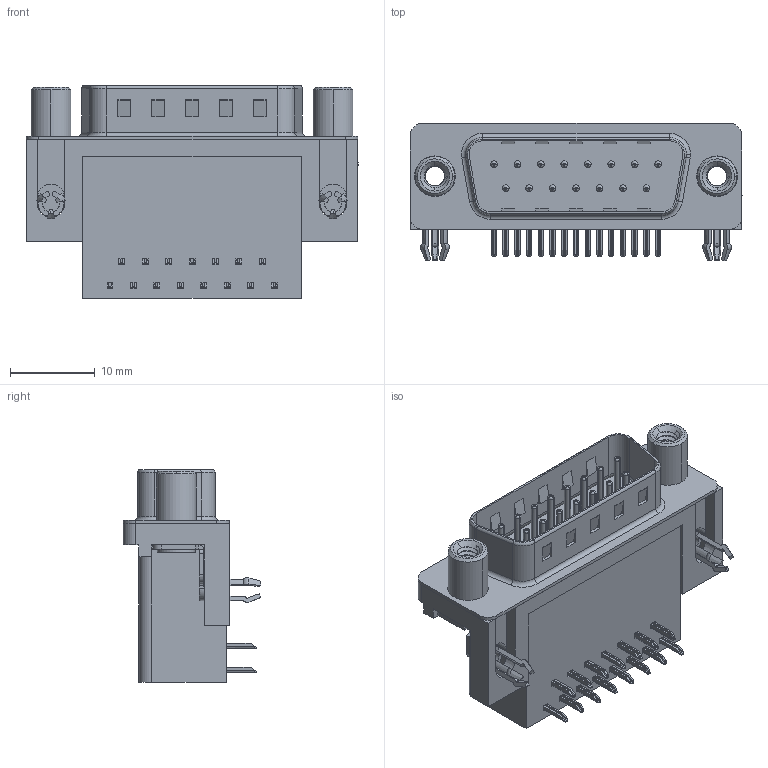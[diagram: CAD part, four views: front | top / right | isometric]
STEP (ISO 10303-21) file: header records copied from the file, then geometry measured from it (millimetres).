
FILE_DESCRIPTION (( 'STEP AP203' ), '1' );
FILE_NAME ('625-015-662-040.STEP', '2018-11-06T00:22:22', ( '' ), ( '' ), 'SwSTEP 2.0', 'SolidWorks 2016', '' );
FILE_SCHEMA (( 'CONFIG_CONTROL_DESIGN' ));
Length unit declared in the file: millimetre
Products named in the file (7): 625 Contact Bottom; 625 Contact Top; 625 3 Prong Board Lock; 625 Round Threaded Standoff; 625-015-662-040; 625 Housing_15 Socket; 625 Shell_15 Socket
Assembly tree (21 placements, depth 2):
  625-015-662-040
    625 Housing_15 Socket
    625 Shell_15 Socket
    625 Contact Bottom  x7
    625 Contact Top  x8
    625 3 Prong Board Lock  x2
    625 Round Threaded Standoff  x2
Bounding box: 39.22 x 16.25 x 25.16 mm (x, y, z)
Volume: 6341.7 mm3; surface area: 6684.6 mm2
Topology: 21 solids, 21 shells, 1577 faces, 3991 edges, 2491 vertices
Faces by surface type: plane 923, cylinder 461, torus 129, cone 48, bspline 16
Entity records: 20897 total; most frequent: CARTESIAN_POINT 5069, DIRECTION 3114, ORIENTED_EDGE 3024, EDGE_CURVE 1512, AXIS2_PLACEMENT_3D 1060, LINE 994, VECTOR 994, VERTEX_POINT 971
